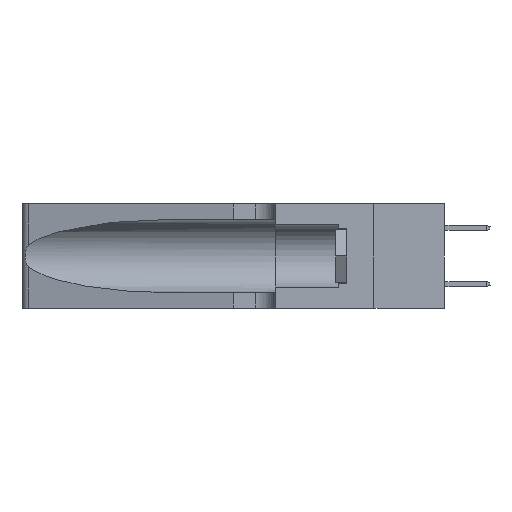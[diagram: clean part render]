
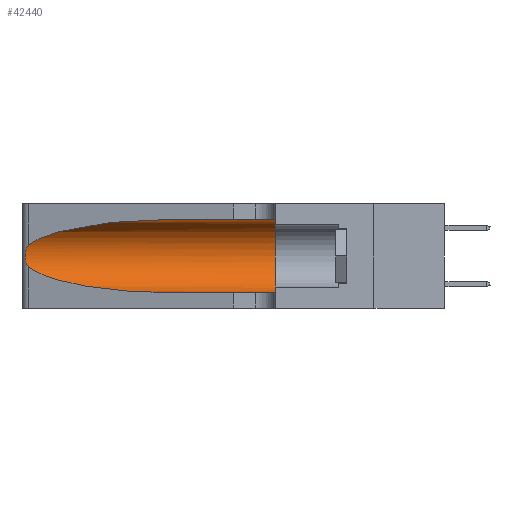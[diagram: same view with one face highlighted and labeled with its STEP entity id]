
A CAD part, left-side view. The second image highlights one B-rep face of the part: STEP entity #42440.
In plain terms, the highlighted cylindrical face has radius 3.308 mm (diameter 6.617 mm), a partial arc.
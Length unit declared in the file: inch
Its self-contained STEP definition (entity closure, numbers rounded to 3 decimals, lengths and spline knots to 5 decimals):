
#980 = LINE ( 'NONE', #6020, #17817 ) ;
#1647 = CARTESIAN_POINT ( 'NONE',  ( 0.25789, 1.23486, 0.15765 ) ) ;
#2142 = ORIENTED_EDGE ( 'NONE', *, *, #23699, .T. ) ;
#2274 = CARTESIAN_POINT ( 'NONE',  ( 0.26075, 1.23896, 0.19203 ) ) ;
#2929 = CARTESIAN_POINT ( 'NONE',  ( 0.1305, 0.35, 0.185 ) ) ;
#4261 = AXIS2_PLACEMENT_3D ( 'NONE', #2929, #14893, #39624 ) ;
#4267 = CARTESIAN_POINT ( 'NONE',  ( 0.25487, 1.22718, 0.22369 ) ) ;
#4334 = CYLINDRICAL_SURFACE ( 'NONE', #15930, 0.13025 ) ;
#5470 = CARTESIAN_POINT ( 'NONE',  ( 0.26018, 1.23835, 0.19895 ) ) ;
#5583 = EDGE_CURVE ( 'NONE', #40610, #33035, #27190, .T. ) ;
#5617 = CARTESIAN_POINT ( 'NONE',  ( 0.26017, 1.23833, 0.17102 ) ) ;
#6020 = CARTESIAN_POINT ( 'NONE',  ( 0.1305, 1.61858, 0.05475 ) ) ;
#8435 = EDGE_LOOP ( 'NONE', ( #40815, #2142, #34988, #43154, #10955, #36526 ) ) ;
#9356 = CARTESIAN_POINT ( 'NONE',  ( 0.25555, 1.22994, 0.2215 ) ) ;
#9531 = DIRECTION ( 'NONE',  ( 0., -1., 0. ) ) ;
#10226 = CARTESIAN_POINT ( 'NONE',  ( 0.25555, 1.22993, 0.14849 ) ) ;
#10253 = CARTESIAN_POINT ( 'NONE',  ( 0.25854, 1.2359, 0.20912 ) ) ;
#10955 = ORIENTED_EDGE ( 'NONE', *, *, #19925, .F. ) ;
#11093 = CARTESIAN_POINT ( 'NONE',  ( 0.1305, 0.72297, 0.05475 ) ) ;
#11561 = B_SPLINE_CURVE_WITH_KNOTS ( 'NONE', 3,
 ( #4267, #9356, #26675, #25942, #10253, #5470, #2274, #15472, #5617, #43869, #1647, #24186, #10226, #44586 ),
 .UNSPECIFIED., .F., .F.,
 ( 4, 2, 2, 2, 2, 2, 4 ),
 ( 0., 0.00027, 0.00053, 0.00107, 0.0016, 0.00187, 0.00214 ),
 .UNSPECIFIED. ) ;
#13289 = CARTESIAN_POINT ( 'NONE',  ( 0.1305, 0.72297, 0.31525 ) ) ;
#14893 = DIRECTION ( 'NONE',  ( 0., 1., 0. ) ) ;
#15151 = DIRECTION ( 'NONE',  ( 0., 0., -1. ) ) ;
#15472 = CARTESIAN_POINT ( 'NONE',  ( 0.26075, 1.23896, 0.178 ) ) ;
#15930 = AXIS2_PLACEMENT_3D ( 'NONE', #25792, #36410, #15151 ) ;
#16741 = VECTOR ( 'NONE', #9531, 39.37008 ) ;
#17757 = CARTESIAN_POINT ( 'NONE',  ( 0.25487, 1.22718, 0.14631 ) ) ;
#17817 = VECTOR ( 'NONE', #40919, 39.37008 ) ;
#17906 = CARTESIAN_POINT ( 'NONE',  ( 0.2373, 1.15595, 0.28018 ) ) ;
#18306 = CARTESIAN_POINT ( 'NONE',  ( 0.1305, 0.35, 0.31525 ) ) ;
#19464 = EDGE_CURVE ( 'NONE', #24624, #23870, #29854, .T. ) ;
#19925 = EDGE_CURVE ( 'NONE', #23870, #39601, #34662, .T. ) ;
#23360 = CARTESIAN_POINT ( 'NONE',  ( 0.1305, 1.61858, 0.31525 ) ) ;
#23699 = EDGE_CURVE ( 'NONE', #26612, #40610, #11561, .T. ) ;
#23870 = VERTEX_POINT ( 'NONE', #18306 ) ;
#24186 = CARTESIAN_POINT ( 'NONE',  ( 0.25639, 1.23186, 0.15144 ) ) ;
#24624 = VERTEX_POINT ( 'NONE', #32522 ) ;
#25792 = CARTESIAN_POINT ( 'NONE',  ( 0.1305, 1.61858, 0.185 ) ) ;
#25942 = CARTESIAN_POINT ( 'NONE',  ( 0.25787, 1.23484, 0.2124 ) ) ;
#26612 = VERTEX_POINT ( 'NONE', #33915 ) ;
#26675 = CARTESIAN_POINT ( 'NONE',  ( 0.25639, 1.23184, 0.21858 ) ) ;
#26686 = EDGE_CURVE ( 'NONE', #24624, #26612, #29975, .T. ) ;
#27190 =( BOUNDED_CURVE ( )  B_SPLINE_CURVE ( 3, ( #17757, #28441, #41925, #11093 ),
 .UNSPECIFIED., .F., .F. ) 
 B_SPLINE_CURVE_WITH_KNOTS ( ( 4, 4 ),
 ( 3.44316, 4.71239 ),
 .UNSPECIFIED. ) 
 CURVE ( )  GEOMETRIC_REPRESENTATION_ITEM ( )  RATIONAL_B_SPLINE_CURVE ( ( 1., 0.87, 0.87, 1. ) ) 
 REPRESENTATION_ITEM ( '' )  );
#28441 = CARTESIAN_POINT ( 'NONE',  ( 0.2373, 1.15595, 0.08982 ) ) ;
#29854 = LINE ( 'NONE', #23360, #16741 ) ;
#29975 =( BOUNDED_CURVE ( )  B_SPLINE_CURVE ( 3, ( #13289, #41017, #17906, #41914 ),
 .UNSPECIFIED., .F., .T. ) 
 B_SPLINE_CURVE_WITH_KNOTS ( ( 4, 4 ),
 ( 1.5708, 2.84003 ),
 .UNSPECIFIED. ) 
 CURVE ( )  GEOMETRIC_REPRESENTATION_ITEM ( )  RATIONAL_B_SPLINE_CURVE ( ( 1., 0.87, 0.87, 1. ) ) 
 REPRESENTATION_ITEM ( '' )  );
#30077 = CARTESIAN_POINT ( 'NONE',  ( 0.25487, 1.22718, 0.14631 ) ) ;
#31448 = CARTESIAN_POINT ( 'NONE',  ( 0.1305, 0.35, 0.05475 ) ) ;
#32522 = CARTESIAN_POINT ( 'NONE',  ( 0.1305, 0.72297, 0.31525 ) ) ;
#33035 = VERTEX_POINT ( 'NONE', #40690 ) ;
#33915 = CARTESIAN_POINT ( 'NONE',  ( 0.25487, 1.22718, 0.22369 ) ) ;
#34662 = CIRCLE ( 'NONE', #4261, 0.13025 ) ;
#34988 = ORIENTED_EDGE ( 'NONE', *, *, #5583, .T. ) ;
#36410 = DIRECTION ( 'NONE',  ( 0., -1., 0. ) ) ;
#36526 = ORIENTED_EDGE ( 'NONE', *, *, #19464, .F. ) ;
#36803 = EDGE_CURVE ( 'NONE', #33035, #39601, #980, .T. ) ;
#39601 = VERTEX_POINT ( 'NONE', #31448 ) ;
#39624 = DIRECTION ( 'NONE',  ( 0., 0., 1. ) ) ;
#40610 = VERTEX_POINT ( 'NONE', #30077 ) ;
#40690 = CARTESIAN_POINT ( 'NONE',  ( 0.1305, 0.72297, 0.05475 ) ) ;
#40708 = FACE_OUTER_BOUND ( 'NONE', #8435, .T. ) ;
#40815 = ORIENTED_EDGE ( 'NONE', *, *, #26686, .T. ) ;
#40919 = DIRECTION ( 'NONE',  ( 0., -1., 0. ) ) ;
#41017 = CARTESIAN_POINT ( 'NONE',  ( 0.18966, 0.96281, 0.31525 ) ) ;
#41914 = CARTESIAN_POINT ( 'NONE',  ( 0.25487, 1.22718, 0.22369 ) ) ;
#41925 = CARTESIAN_POINT ( 'NONE',  ( 0.18966, 0.96281, 0.05475 ) ) ;
#42440 = ADVANCED_FACE ( 'NONE', ( #40708 ), #4334, .F. ) ;
#43154 = ORIENTED_EDGE ( 'NONE', *, *, #36803, .T. ) ;
#43869 = CARTESIAN_POINT ( 'NONE',  ( 0.25856, 1.23593, 0.16098 ) ) ;
#44586 = CARTESIAN_POINT ( 'NONE',  ( 0.25487, 1.22718, 0.14631 ) ) ;
